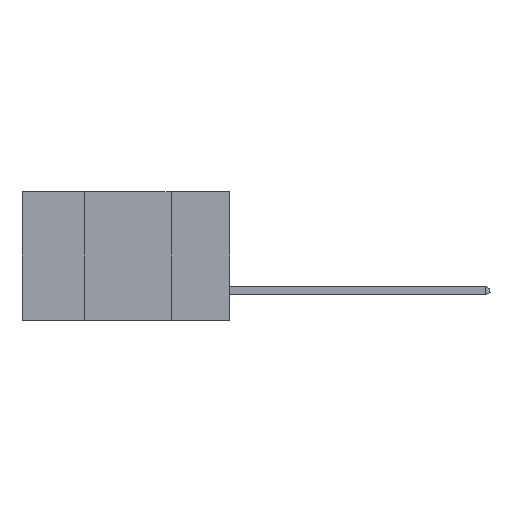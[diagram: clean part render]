
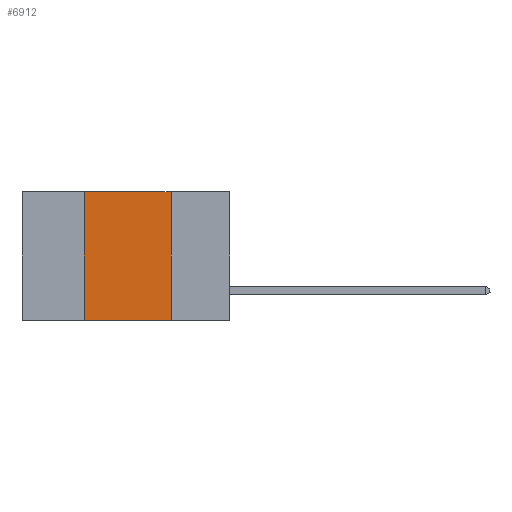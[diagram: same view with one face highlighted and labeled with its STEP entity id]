
A CAD part, left-side view. The second image highlights one B-rep face of the part: STEP entity #6912.
In plain terms, the highlighted planar face has unit normal (-1, 0, 0).
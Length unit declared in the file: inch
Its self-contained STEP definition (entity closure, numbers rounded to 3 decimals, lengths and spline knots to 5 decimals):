
#833 = CARTESIAN_POINT ( 'NONE',  ( 0., 0.6, 0. ) ) ;
#907 = DIRECTION ( 'NONE',  ( 0., -1., 0. ) ) ;
#1581 = VERTEX_POINT ( 'NONE', #9260 ) ;
#1625 = CARTESIAN_POINT ( 'NONE',  ( 0., 0.6, 0. ) ) ;
#1964 = LINE ( 'NONE', #12894, #15162 ) ;
#3125 = VERTEX_POINT ( 'NONE', #6542 ) ;
#3562 = CARTESIAN_POINT ( 'NONE',  ( 0., 0.42, 0. ) ) ;
#4817 = EDGE_LOOP ( 'NONE', ( #15759, #21924, #14113, #18714 ) ) ;
#6531 = EDGE_CURVE ( 'NONE', #22293, #3125, #14004, .T. ) ;
#6542 = CARTESIAN_POINT ( 'NONE',  ( 0., 0.17, -0.37 ) ) ;
#6912 = ADVANCED_FACE ( 'NONE', ( #18398 ), #15437, .F. ) ;
#7465 = DIRECTION ( 'NONE',  ( 0., -1., 0. ) ) ;
#9260 = CARTESIAN_POINT ( 'NONE',  ( 0., 0.42, -0.37 ) ) ;
#9443 = AXIS2_PLACEMENT_3D ( 'NONE', #1625, #13946, #10244 ) ;
#9973 = VERTEX_POINT ( 'NONE', #3562 ) ;
#10244 = DIRECTION ( 'NONE',  ( 0., 0., -1. ) ) ;
#10517 = DIRECTION ( 'NONE',  ( 0., 0., 1. ) ) ;
#10760 = EDGE_CURVE ( 'NONE', #1581, #3125, #1964, .T. ) ;
#10836 = VECTOR ( 'NONE', #10517, 39.37008 ) ;
#11013 = CARTESIAN_POINT ( 'NONE',  ( 0., 0.17, 0. ) ) ;
#12894 = CARTESIAN_POINT ( 'NONE',  ( 0., 0.6, -0.37 ) ) ;
#13490 = EDGE_CURVE ( 'NONE', #9973, #22293, #17991, .T. ) ;
#13716 = EDGE_CURVE ( 'NONE', #1581, #9973, #14940, .T. ) ;
#13946 = DIRECTION ( 'NONE',  ( 1., 0., 0. ) ) ;
#14004 = LINE ( 'NONE', #17964, #15607 ) ;
#14113 = ORIENTED_EDGE ( 'NONE', *, *, #13716, .F. ) ;
#14940 = LINE ( 'NONE', #19135, #10836 ) ;
#15162 = VECTOR ( 'NONE', #7465, 39.37008 ) ;
#15437 = PLANE ( 'NONE',  #9443 ) ;
#15607 = VECTOR ( 'NONE', #21303, 39.37008 ) ;
#15759 = ORIENTED_EDGE ( 'NONE', *, *, #6531, .F. ) ;
#16050 = VECTOR ( 'NONE', #907, 39.37008 ) ;
#17964 = CARTESIAN_POINT ( 'NONE',  ( 0., 0.17, 0. ) ) ;
#17991 = LINE ( 'NONE', #833, #16050 ) ;
#18398 = FACE_OUTER_BOUND ( 'NONE', #4817, .T. ) ;
#18714 = ORIENTED_EDGE ( 'NONE', *, *, #10760, .T. ) ;
#19135 = CARTESIAN_POINT ( 'NONE',  ( 0., 0.42, 0. ) ) ;
#21303 = DIRECTION ( 'NONE',  ( 0., 0., -1. ) ) ;
#21924 = ORIENTED_EDGE ( 'NONE', *, *, #13490, .F. ) ;
#22293 = VERTEX_POINT ( 'NONE', #11013 ) ;
